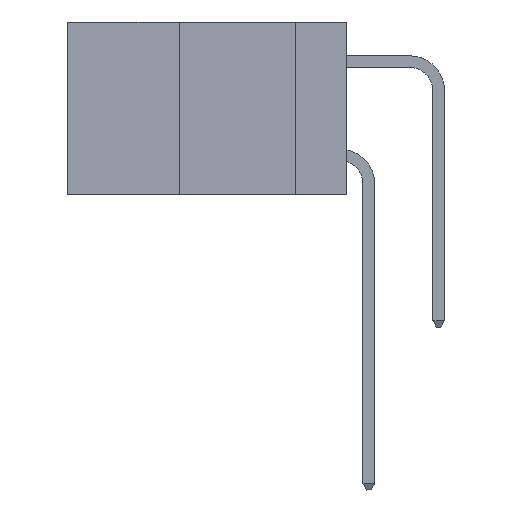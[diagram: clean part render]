
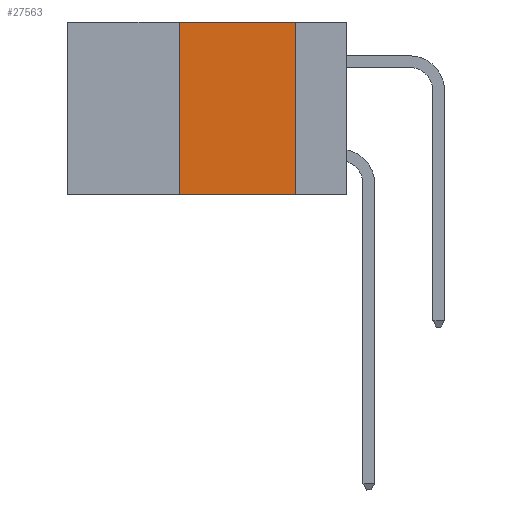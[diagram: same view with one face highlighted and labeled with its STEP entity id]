
A CAD part, left-side view. The second image highlights one B-rep face of the part: STEP entity #27563.
In plain terms, the highlighted planar face has unit normal (-1, 0, 0).
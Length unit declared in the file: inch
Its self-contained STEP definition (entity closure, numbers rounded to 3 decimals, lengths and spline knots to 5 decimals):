
#467 = PLANE ( 'NONE',  #4109 ) ;
#705 = DIRECTION ( 'NONE',  ( 1., 0., 0. ) ) ;
#3355 = DIRECTION ( 'NONE',  ( 0., -1., 0. ) ) ;
#4109 = AXIS2_PLACEMENT_3D ( 'NONE', #33598, #705, #6324 ) ;
#4328 = CARTESIAN_POINT ( 'NONE',  ( 0., 0.11, 0. ) ) ;
#4697 = CARTESIAN_POINT ( 'NONE',  ( 0., 0.36, 0. ) ) ;
#4741 = ORIENTED_EDGE ( 'NONE', *, *, #33446, .F. ) ;
#6324 = DIRECTION ( 'NONE',  ( 0., 0., -1. ) ) ;
#7295 = LINE ( 'NONE', #21873, #27767 ) ;
#8047 = CARTESIAN_POINT ( 'NONE',  ( 0., 0.6, -0.37 ) ) ;
#9748 = EDGE_CURVE ( 'NONE', #21548, #21356, #10360, .T. ) ;
#10360 = LINE ( 'NONE', #27407, #34284 ) ;
#11667 = EDGE_CURVE ( 'NONE', #17049, #15841, #24587, .T. ) ;
#11909 = CARTESIAN_POINT ( 'NONE',  ( 0., 0.36, -0.37 ) ) ;
#13760 = FACE_OUTER_BOUND ( 'NONE', #34690, .T. ) ;
#15469 = VECTOR ( 'NONE', #31709, 39.37008 ) ;
#15841 = VERTEX_POINT ( 'NONE', #4697 ) ;
#16017 = LINE ( 'NONE', #8047, #24237 ) ;
#17049 = VERTEX_POINT ( 'NONE', #11909 ) ;
#19237 = DIRECTION ( 'NONE',  ( 0., -1., 0. ) ) ;
#20619 = CARTESIAN_POINT ( 'NONE',  ( 0., 0.36, 0. ) ) ;
#21356 = VERTEX_POINT ( 'NONE', #28597 ) ;
#21548 = VERTEX_POINT ( 'NONE', #4328 ) ;
#21873 = CARTESIAN_POINT ( 'NONE',  ( 0., 0.6, 0. ) ) ;
#23689 = ORIENTED_EDGE ( 'NONE', *, *, #11667, .F. ) ;
#24237 = VECTOR ( 'NONE', #19237, 39.37008 ) ;
#24587 = LINE ( 'NONE', #20619, #15469 ) ;
#25533 = EDGE_CURVE ( 'NONE', #17049, #21356, #16017, .T. ) ;
#26988 = ORIENTED_EDGE ( 'NONE', *, *, #9748, .F. ) ;
#27407 = CARTESIAN_POINT ( 'NONE',  ( 0., 0.11, 0. ) ) ;
#27563 = ADVANCED_FACE ( 'NONE', ( #13760 ), #467, .F. ) ;
#27767 = VECTOR ( 'NONE', #3355, 39.37008 ) ;
#28597 = CARTESIAN_POINT ( 'NONE',  ( 0., 0.11, -0.37 ) ) ;
#31709 = DIRECTION ( 'NONE',  ( 0., 0., 1. ) ) ;
#33365 = DIRECTION ( 'NONE',  ( 0., 0., -1. ) ) ;
#33446 = EDGE_CURVE ( 'NONE', #15841, #21548, #7295, .T. ) ;
#33598 = CARTESIAN_POINT ( 'NONE',  ( 0., 0.6, 0. ) ) ;
#34284 = VECTOR ( 'NONE', #33365, 39.37008 ) ;
#34690 = EDGE_LOOP ( 'NONE', ( #26988, #4741, #23689, #35166 ) ) ;
#35166 = ORIENTED_EDGE ( 'NONE', *, *, #25533, .T. ) ;
